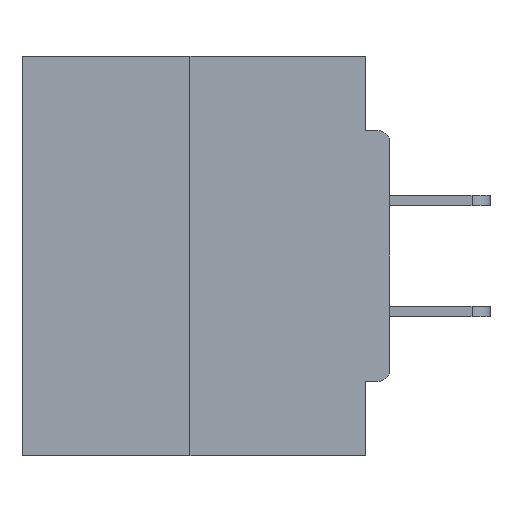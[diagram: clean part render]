
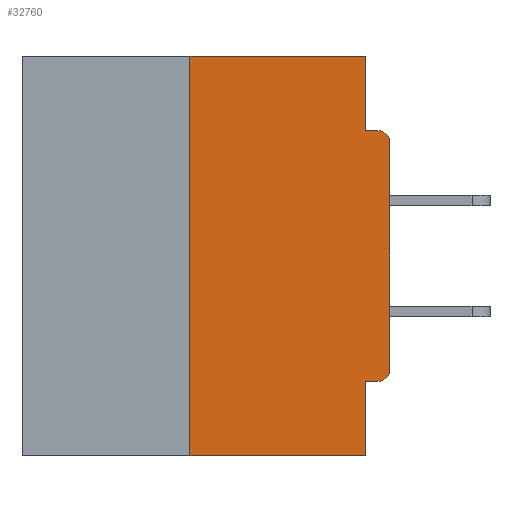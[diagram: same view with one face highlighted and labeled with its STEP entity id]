
A CAD part, left-side view. The second image highlights one B-rep face of the part: STEP entity #32760.
In plain terms, the highlighted planar face has unit normal (-1, 0, 0).
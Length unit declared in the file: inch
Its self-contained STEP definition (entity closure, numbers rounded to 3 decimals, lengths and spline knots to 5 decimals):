
#261 = VERTEX_POINT ( 'NONE', #9540 ) ;
#352 = VECTOR ( 'NONE', #17091, 39.37008 ) ;
#459 = EDGE_CURVE ( 'NONE', #8212, #33352, #1167, .T. ) ;
#722 = DIRECTION ( 'NONE',  ( 0., 1., 0. ) ) ;
#1167 = LINE ( 'NONE', #7134, #28679 ) ;
#1427 = EDGE_CURVE ( 'NONE', #7847, #8212, #21621, .T. ) ;
#2206 = CARTESIAN_POINT ( 'NONE',  ( 0., 0.031, -0.0935 ) ) ;
#3032 = DIRECTION ( 'NONE',  ( 0., 0., -1. ) ) ;
#3465 = VERTEX_POINT ( 'NONE', #20705 ) ;
#3548 = VERTEX_POINT ( 'NONE', #3686 ) ;
#3646 = PLANE ( 'NONE',  #23827 ) ;
#3686 = CARTESIAN_POINT ( 'NONE',  ( 0., 0.25, -0.5 ) ) ;
#3893 = VECTOR ( 'NONE', #722, 39.37008 ) ;
#4118 = CARTESIAN_POINT ( 'NONE',  ( 0., 0., 0. ) ) ;
#4191 = CARTESIAN_POINT ( 'NONE',  ( 0., 0.25, 0. ) ) ;
#4506 = ORIENTED_EDGE ( 'NONE', *, *, #10134, .T. ) ;
#4560 = LINE ( 'NONE', #15961, #15056 ) ;
#5787 = DIRECTION ( 'NONE',  ( 0., 0., -1. ) ) ;
#6015 = CARTESIAN_POINT ( 'NONE',  ( 0., 0.015, -0.1085 ) ) ;
#6483 = ORIENTED_EDGE ( 'NONE', *, *, #20075, .F. ) ;
#6683 = ORIENTED_EDGE ( 'NONE', *, *, #459, .F. ) ;
#7035 = DIRECTION ( 'NONE',  ( 0., 0., 1. ) ) ;
#7134 = CARTESIAN_POINT ( 'NONE',  ( 0., 0., -0.0935 ) ) ;
#7311 = CARTESIAN_POINT ( 'NONE',  ( 0., 0.015, -0.0935 ) ) ;
#7466 = VERTEX_POINT ( 'NONE', #17316 ) ;
#7493 = CIRCLE ( 'NONE', #14963, 0.015 ) ;
#7609 = CARTESIAN_POINT ( 'NONE',  ( 0., 0.015, -0.4065 ) ) ;
#7752 = LINE ( 'NONE', #4118, #29133 ) ;
#7787 = CARTESIAN_POINT ( 'NONE',  ( 0., 0.031, 0. ) ) ;
#7847 = VERTEX_POINT ( 'NONE', #7787 ) ;
#8024 = ORIENTED_EDGE ( 'NONE', *, *, #23552, .F. ) ;
#8212 = VERTEX_POINT ( 'NONE', #2206 ) ;
#8412 = EDGE_CURVE ( 'NONE', #7466, #33352, #35398, .T. ) ;
#8738 = LINE ( 'NONE', #10721, #19191 ) ;
#9540 = CARTESIAN_POINT ( 'NONE',  ( 0., 0.031, -0.4065 ) ) ;
#9859 = EDGE_CURVE ( 'NONE', #261, #3465, #8738, .T. ) ;
#10134 = EDGE_CURVE ( 'NONE', #3548, #3465, #18745, .T. ) ;
#10721 = CARTESIAN_POINT ( 'NONE',  ( 0., 0.031, -0.5 ) ) ;
#10902 = EDGE_CURVE ( 'NONE', #19445, #7466, #7752, .T. ) ;
#11813 = FACE_OUTER_BOUND ( 'NONE', #18941, .T. ) ;
#12208 = DIRECTION ( 'NONE',  ( 0., 0., -1. ) ) ;
#14307 = CARTESIAN_POINT ( 'NONE',  ( 0., 0.46, 0. ) ) ;
#14392 = VERTEX_POINT ( 'NONE', #4191 ) ;
#14404 = DIRECTION ( 'NONE',  ( 0., 0., -1. ) ) ;
#14963 = AXIS2_PLACEMENT_3D ( 'NONE', #31050, #17424, #14404 ) ;
#15056 = VECTOR ( 'NONE', #18799, 39.37008 ) ;
#15961 = CARTESIAN_POINT ( 'NONE',  ( 0., 0.25, 0. ) ) ;
#16855 = VECTOR ( 'NONE', #12208, 39.37008 ) ;
#17091 = DIRECTION ( 'NONE',  ( 0., -1., 0. ) ) ;
#17122 = ORIENTED_EDGE ( 'NONE', *, *, #9859, .F. ) ;
#17316 = CARTESIAN_POINT ( 'NONE',  ( 0., 0., -0.1085 ) ) ;
#17424 = DIRECTION ( 'NONE',  ( -1., 0., 0. ) ) ;
#17443 = LINE ( 'NONE', #17471, #3893 ) ;
#17471 = CARTESIAN_POINT ( 'NONE',  ( 0., 0., -0.4065 ) ) ;
#18745 = LINE ( 'NONE', #30489, #32639 ) ;
#18799 = DIRECTION ( 'NONE',  ( 0., 0., 1. ) ) ;
#18941 = EDGE_LOOP ( 'NONE', ( #19175, #6483, #4506, #17122, #8024, #23697, #25465, #26161, #6683, #34363 ) ) ;
#19175 = ORIENTED_EDGE ( 'NONE', *, *, #33591, .F. ) ;
#19191 = VECTOR ( 'NONE', #3032, 39.37008 ) ;
#19445 = VERTEX_POINT ( 'NONE', #32640 ) ;
#20075 = EDGE_CURVE ( 'NONE', #3548, #14392, #4560, .T. ) ;
#20705 = CARTESIAN_POINT ( 'NONE',  ( 0., 0.031, -0.5 ) ) ;
#21161 = DIRECTION ( 'NONE',  ( 0., -1., 0. ) ) ;
#21295 = EDGE_CURVE ( 'NONE', #36068, #19445, #7493, .T. ) ;
#21621 = LINE ( 'NONE', #23745, #16855 ) ;
#22650 = LINE ( 'NONE', #14307, #352 ) ;
#22920 = DIRECTION ( 'NONE',  ( 0., 0., -1. ) ) ;
#23552 = EDGE_CURVE ( 'NONE', #36068, #261, #17443, .T. ) ;
#23697 = ORIENTED_EDGE ( 'NONE', *, *, #21295, .T. ) ;
#23745 = CARTESIAN_POINT ( 'NONE',  ( 0., 0.031, 0. ) ) ;
#23827 = AXIS2_PLACEMENT_3D ( 'NONE', #26200, #31322, #22920 ) ;
#25465 = ORIENTED_EDGE ( 'NONE', *, *, #10902, .T. ) ;
#26161 = ORIENTED_EDGE ( 'NONE', *, *, #8412, .T. ) ;
#26200 = CARTESIAN_POINT ( 'NONE',  ( 0., 0.46, 0. ) ) ;
#28073 = AXIS2_PLACEMENT_3D ( 'NONE', #6015, #31371, #5787 ) ;
#28679 = VECTOR ( 'NONE', #21161, 39.37008 ) ;
#29133 = VECTOR ( 'NONE', #7035, 39.37008 ) ;
#30489 = CARTESIAN_POINT ( 'NONE',  ( 0., 0.46, -0.5 ) ) ;
#31050 = CARTESIAN_POINT ( 'NONE',  ( 0., 0.015, -0.3915 ) ) ;
#31322 = DIRECTION ( 'NONE',  ( 1., 0., 0. ) ) ;
#31371 = DIRECTION ( 'NONE',  ( -1., 0., 0. ) ) ;
#32639 = VECTOR ( 'NONE', #35725, 39.37008 ) ;
#32640 = CARTESIAN_POINT ( 'NONE',  ( 0., 0., -0.3915 ) ) ;
#32760 = ADVANCED_FACE ( 'NONE', ( #11813 ), #3646, .F. ) ;
#33352 = VERTEX_POINT ( 'NONE', #7311 ) ;
#33591 = EDGE_CURVE ( 'NONE', #14392, #7847, #22650, .T. ) ;
#34363 = ORIENTED_EDGE ( 'NONE', *, *, #1427, .F. ) ;
#35398 = CIRCLE ( 'NONE', #28073, 0.015 ) ;
#35725 = DIRECTION ( 'NONE',  ( 0., -1., 0. ) ) ;
#36068 = VERTEX_POINT ( 'NONE', #7609 ) ;
